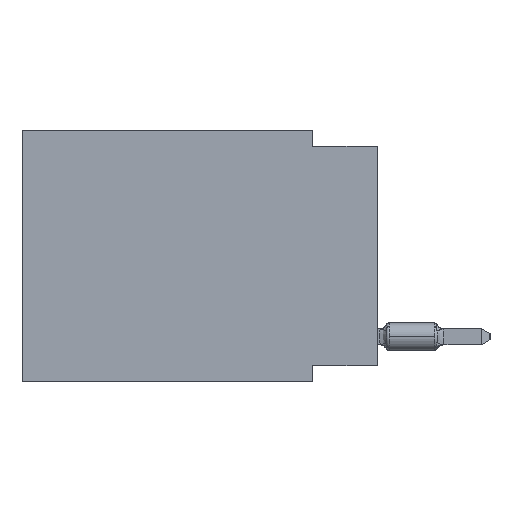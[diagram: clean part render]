
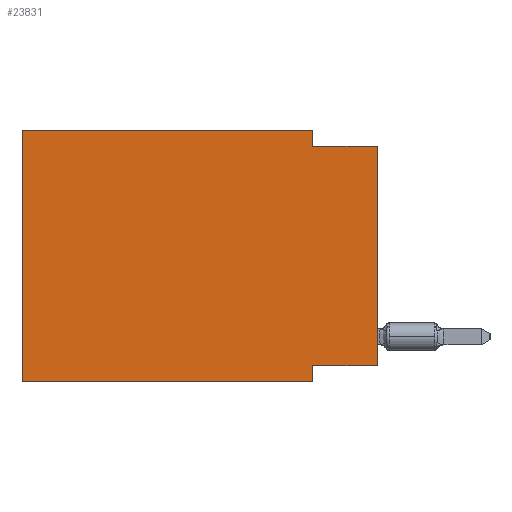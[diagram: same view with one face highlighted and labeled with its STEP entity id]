
A CAD part, left-side view. The second image highlights one B-rep face of the part: STEP entity #23831.
In plain terms, the highlighted planar face has unit normal (-1, 0, 0).
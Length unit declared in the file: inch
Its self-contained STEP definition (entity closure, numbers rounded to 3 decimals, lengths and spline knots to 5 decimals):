
#919 = VECTOR ( 'NONE', #11212, 39.37008 ) ;
#1354 = VERTEX_POINT ( 'NONE', #20560 ) ;
#1377 = CARTESIAN_POINT ( 'NONE',  ( 0., 0.1, -0.39 ) ) ;
#1460 = ORIENTED_EDGE ( 'NONE', *, *, #21969, .T. ) ;
#1660 = CARTESIAN_POINT ( 'NONE',  ( 0., 0., -0.365 ) ) ;
#2310 = LINE ( 'NONE', #10056, #17651 ) ;
#2736 = VERTEX_POINT ( 'NONE', #13807 ) ;
#2895 = DIRECTION ( 'NONE',  ( 0., 0., -1. ) ) ;
#2949 = DIRECTION ( 'NONE',  ( 1., 0., 0. ) ) ;
#3019 = LINE ( 'NONE', #6966, #12343 ) ;
#3314 = CARTESIAN_POINT ( 'NONE',  ( 0., 0.1, -0.025 ) ) ;
#3461 = CARTESIAN_POINT ( 'NONE',  ( 0., 0.55, 0. ) ) ;
#3470 = VERTEX_POINT ( 'NONE', #21096 ) ;
#4868 = CARTESIAN_POINT ( 'NONE',  ( 0., 0.55, 0. ) ) ;
#5497 = EDGE_CURVE ( 'NONE', #3470, #10960, #9455, .T. ) ;
#5869 = EDGE_CURVE ( 'NONE', #14437, #1354, #22774, .T. ) ;
#6049 = ORIENTED_EDGE ( 'NONE', *, *, #19370, .F. ) ;
#6374 = DIRECTION ( 'NONE',  ( 0., -1., 0. ) ) ;
#6966 = CARTESIAN_POINT ( 'NONE',  ( 0., 0., -0.025 ) ) ;
#7211 = DIRECTION ( 'NONE',  ( 0., -1., 0. ) ) ;
#9351 = CARTESIAN_POINT ( 'NONE',  ( 0., 0.55, -0.39 ) ) ;
#9455 = LINE ( 'NONE', #17213, #16687 ) ;
#10056 = CARTESIAN_POINT ( 'NONE',  ( 0., 0.55, 0. ) ) ;
#10222 = CARTESIAN_POINT ( 'NONE',  ( 0., 0.55, -0.39 ) ) ;
#10264 = VERTEX_POINT ( 'NONE', #1660 ) ;
#10471 = DIRECTION ( 'NONE',  ( 0., 0., -1. ) ) ;
#10960 = VERTEX_POINT ( 'NONE', #3314 ) ;
#11107 = AXIS2_PLACEMENT_3D ( 'NONE', #4868, #2949, #10471 ) ;
#11212 = DIRECTION ( 'NONE',  ( 0., 0., 1. ) ) ;
#11442 = ORIENTED_EDGE ( 'NONE', *, *, #5497, .F. ) ;
#12244 = LINE ( 'NONE', #18216, #20815 ) ;
#12343 = VECTOR ( 'NONE', #14701, 39.37008 ) ;
#13276 = ORIENTED_EDGE ( 'NONE', *, *, #13569, .T. ) ;
#13372 = CARTESIAN_POINT ( 'NONE',  ( 0., 0., 0. ) ) ;
#13569 = EDGE_CURVE ( 'NONE', #10264, #2736, #13637, .T. ) ;
#13637 = LINE ( 'NONE', #13372, #15112 ) ;
#13646 = VERTEX_POINT ( 'NONE', #24037 ) ;
#13807 = CARTESIAN_POINT ( 'NONE',  ( 0., 0., -0.025 ) ) ;
#14162 = EDGE_LOOP ( 'NONE', ( #13276, #23275, #11442, #14638, #23409, #1460, #6049, #15809 ) ) ;
#14364 = VECTOR ( 'NONE', #2895, 39.37008 ) ;
#14437 = VERTEX_POINT ( 'NONE', #10222 ) ;
#14638 = ORIENTED_EDGE ( 'NONE', *, *, #16534, .F. ) ;
#14701 = DIRECTION ( 'NONE',  ( 0., -1., 0. ) ) ;
#15112 = VECTOR ( 'NONE', #24944, 39.37008 ) ;
#15809 = ORIENTED_EDGE ( 'NONE', *, *, #22694, .F. ) ;
#16474 = CARTESIAN_POINT ( 'NONE',  ( 0., 0.1, -0.39 ) ) ;
#16534 = EDGE_CURVE ( 'NONE', #1354, #3470, #2310, .T. ) ;
#16687 = VECTOR ( 'NONE', #24980, 39.37008 ) ;
#17070 = VERTEX_POINT ( 'NONE', #16474 ) ;
#17213 = CARTESIAN_POINT ( 'NONE',  ( 0., 0.1, 0. ) ) ;
#17651 = VECTOR ( 'NONE', #6374, 39.37008 ) ;
#18216 = CARTESIAN_POINT ( 'NONE',  ( 0., 0., -0.365 ) ) ;
#18367 = VECTOR ( 'NONE', #7211, 39.37008 ) ;
#18781 = LINE ( 'NONE', #1377, #14364 ) ;
#19242 = EDGE_CURVE ( 'NONE', #10960, #2736, #3019, .T. ) ;
#19370 = EDGE_CURVE ( 'NONE', #13646, #17070, #18781, .T. ) ;
#19999 = DIRECTION ( 'NONE',  ( 0., 1., 0. ) ) ;
#20365 = FACE_OUTER_BOUND ( 'NONE', #14162, .T. ) ;
#20560 = CARTESIAN_POINT ( 'NONE',  ( 0., 0.55, 0. ) ) ;
#20815 = VECTOR ( 'NONE', #19999, 39.37008 ) ;
#21096 = CARTESIAN_POINT ( 'NONE',  ( 0., 0.1, 0. ) ) ;
#21969 = EDGE_CURVE ( 'NONE', #14437, #17070, #24627, .T. ) ;
#22285 = PLANE ( 'NONE',  #11107 ) ;
#22694 = EDGE_CURVE ( 'NONE', #10264, #13646, #12244, .T. ) ;
#22774 = LINE ( 'NONE', #3461, #919 ) ;
#23275 = ORIENTED_EDGE ( 'NONE', *, *, #19242, .F. ) ;
#23409 = ORIENTED_EDGE ( 'NONE', *, *, #5869, .F. ) ;
#23831 = ADVANCED_FACE ( 'NONE', ( #20365 ), #22285, .F. ) ;
#24037 = CARTESIAN_POINT ( 'NONE',  ( 0., 0.1, -0.365 ) ) ;
#24627 = LINE ( 'NONE', #9351, #18367 ) ;
#24944 = DIRECTION ( 'NONE',  ( 0., 0., 1. ) ) ;
#24980 = DIRECTION ( 'NONE',  ( 0., 0., -1. ) ) ;
